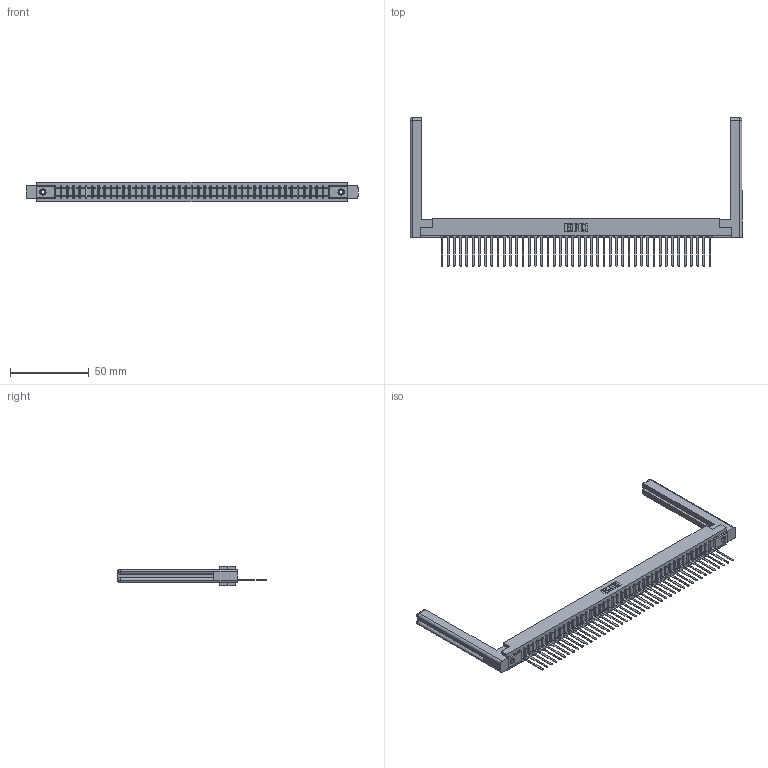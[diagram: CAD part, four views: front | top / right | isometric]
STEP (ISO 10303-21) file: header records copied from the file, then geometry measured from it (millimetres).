
FILE_DESCRIPTION (( 'STEP AP203' ), '1' );
FILE_NAME ('307-044-545-158.STEP', '2019-09-04T11:13:23', ( '' ), ( '' ), 'SwSTEP 2.0', 'SolidWorks 2016', '' );
FILE_SCHEMA (( 'CONFIG_CONTROL_DESIGN' ));
Length unit declared in the file: inch
Products named in the file (5): 307-290-001_545; 345-250-001_345-250-001-102; 307-044-545-158; 307 Part_.156 Dia Mounting Holes; 307-220-058
Assembly tree (49 placements, depth 2):
  307-044-545-158
    307 Part_.156 Dia Mounting Holes
    307-290-001_545  x44
    307-220-058  x2
    345-250-001_345-250-001-102  x2
Bounding box: 210.97 x 94.31 x 12.7 mm (x, y, z)
Volume: 29256 mm3; surface area: 29747.8 mm2
Topology: 49 solids, 49 shells, 2769 faces, 7805 edges, 5010 vertices
Faces by surface type: plane 1782, cylinder 873, sphere 90, torus 12, cone 12
Entity records: 40075 total; most frequent: CARTESIAN_POINT 6759, ORIENTED_EDGE 6684, DIRECTION 6532, EDGE_CURVE 3342, LINE 2562, VECTOR 2562, VERTEX_POINT 2158, AXIS2_PLACEMENT_3D 1985
